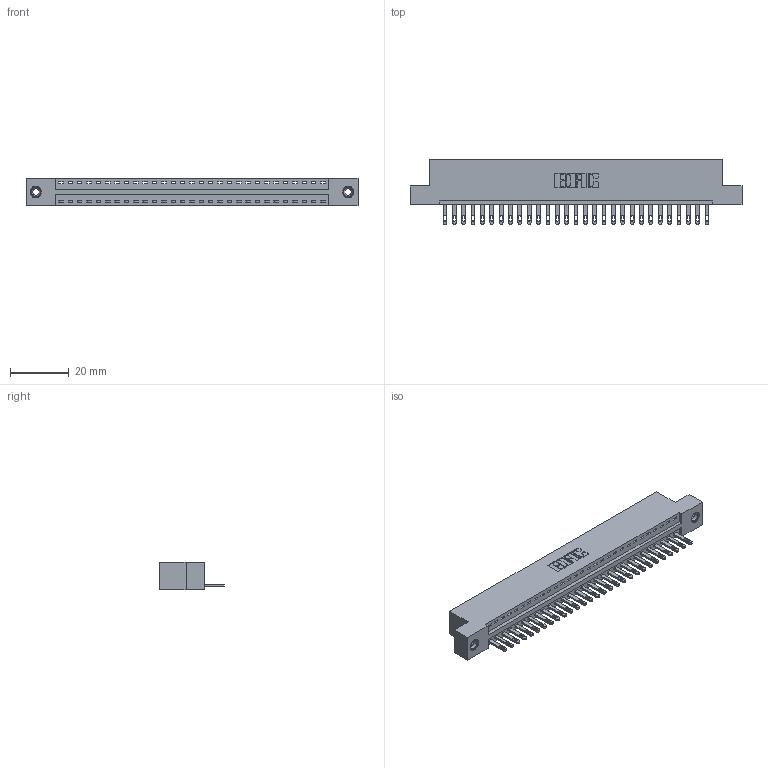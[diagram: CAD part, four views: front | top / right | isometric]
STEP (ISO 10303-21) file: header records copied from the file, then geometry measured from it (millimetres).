
FILE_DESCRIPTION (( 'STEP AP203' ), '1' );
FILE_NAME ('896-029-500-108.STEP', '2021-07-27T18:35:05', ( '' ), ( '' ), 'SwSTEP 2.0', 'SolidWorks 2020', '' );
FILE_SCHEMA (( 'CONFIG_CONTROL_DESIGN' ));
Length unit declared in the file: inch
Products named in the file (4): 345-292-001_345-293-100; 846 Part_Flush Mounting Lugs - 0.156 Dia-TI; 345-250-001_345-250-003-102; 896-029-500-108
Assembly tree (32 placements, depth 2):
  896-029-500-108
    846 Part_Flush Mounting Lugs - 0.156 Dia-TI
    345-292-001_345-293-100  x29
    345-250-001_345-250-003-102  x2
Bounding box: 112.65 x 21.84 x 9.4 mm (x, y, z)
Volume: 10704.9 mm3; surface area: 13328.8 mm2
Topology: 32 solids, 32 shells, 1748 faces, 5337 edges, 3550 vertices
Faces by surface type: plane 1094, cylinder 638, cone 12, torus 4
Entity records: 20864 total; most frequent: CARTESIAN_POINT 3562, ORIENTED_EDGE 3518, DIRECTION 3187, EDGE_CURVE 1759, LINE 1487, VECTOR 1487, VERTEX_POINT 1168, AXIS2_PLACEMENT_3D 850
